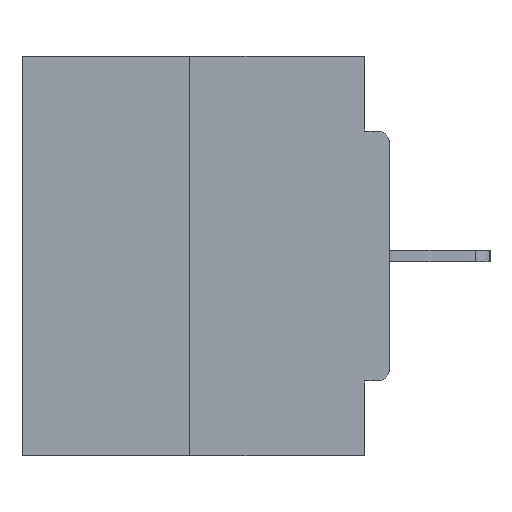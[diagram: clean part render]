
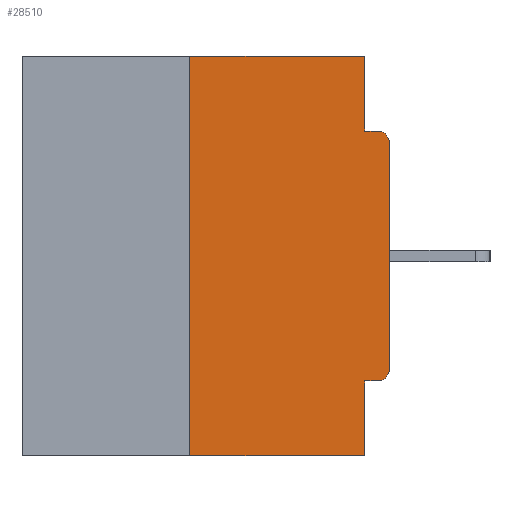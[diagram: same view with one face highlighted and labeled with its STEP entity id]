
A CAD part, left-side view. The second image highlights one B-rep face of the part: STEP entity #28510.
In plain terms, the highlighted planar face has unit normal (-1, 0, 0).
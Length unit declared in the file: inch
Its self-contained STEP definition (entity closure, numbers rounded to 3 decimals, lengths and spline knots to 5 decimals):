
#132 = EDGE_CURVE ( 'NONE', #11339, #19578, #5779, .T. ) ;
#940 = LINE ( 'NONE', #21216, #10678 ) ;
#1049 = LINE ( 'NONE', #2670, #8321 ) ;
#1246 = CARTESIAN_POINT ( 'NONE',  ( 0., 0.015, -0.3915 ) ) ;
#1707 = VECTOR ( 'NONE', #6187, 39.37008 ) ;
#2293 = CARTESIAN_POINT ( 'NONE',  ( 0., 0.25, 0. ) ) ;
#2670 = CARTESIAN_POINT ( 'NONE',  ( 0., 0.25, 0. ) ) ;
#2847 = CARTESIAN_POINT ( 'NONE',  ( 0., 0.015, -0.4065 ) ) ;
#2903 = DIRECTION ( 'NONE',  ( 0., 0., 1. ) ) ;
#3135 = EDGE_CURVE ( 'NONE', #23042, #11339, #20975, .T. ) ;
#3636 = CARTESIAN_POINT ( 'NONE',  ( 0., 0.031, -0.5 ) ) ;
#3715 = CARTESIAN_POINT ( 'NONE',  ( 0., 0.031, 0. ) ) ;
#3979 = ORIENTED_EDGE ( 'NONE', *, *, #6966, .F. ) ;
#4812 = ORIENTED_EDGE ( 'NONE', *, *, #18256, .F. ) ;
#4814 = AXIS2_PLACEMENT_3D ( 'NONE', #7182, #20395, #8969 ) ;
#4815 = CARTESIAN_POINT ( 'NONE',  ( 0., 0.46, 0. ) ) ;
#5355 = DIRECTION ( 'NONE',  ( 0., -1., 0. ) ) ;
#5382 = CARTESIAN_POINT ( 'NONE',  ( 0., 0.46, 0. ) ) ;
#5404 = DIRECTION ( 'NONE',  ( 0., 0., -1. ) ) ;
#5779 = CIRCLE ( 'NONE', #4814, 0.015 ) ;
#6086 = CARTESIAN_POINT ( 'NONE',  ( 0., 0.015, -0.0935 ) ) ;
#6166 = ORIENTED_EDGE ( 'NONE', *, *, #13584, .F. ) ;
#6187 = DIRECTION ( 'NONE',  ( 0., 1., 0. ) ) ;
#6230 = DIRECTION ( 'NONE',  ( 0., 0., -1. ) ) ;
#6966 = EDGE_CURVE ( 'NONE', #11009, #18217, #10561, .T. ) ;
#7108 = CARTESIAN_POINT ( 'NONE',  ( 0., 0.031, -0.0935 ) ) ;
#7182 = CARTESIAN_POINT ( 'NONE',  ( 0., 0.015, -0.1085 ) ) ;
#7282 = VECTOR ( 'NONE', #6230, 39.37008 ) ;
#7327 = FACE_OUTER_BOUND ( 'NONE', #16101, .T. ) ;
#8101 = ORIENTED_EDGE ( 'NONE', *, *, #21871, .T. ) ;
#8168 = ORIENTED_EDGE ( 'NONE', *, *, #21212, .F. ) ;
#8279 = VECTOR ( 'NONE', #24406, 39.37008 ) ;
#8321 = VECTOR ( 'NONE', #22941, 39.37008 ) ;
#8373 = AXIS2_PLACEMENT_3D ( 'NONE', #4815, #16277, #5404 ) ;
#8969 = DIRECTION ( 'NONE',  ( 0., 0., -1. ) ) ;
#10210 = CARTESIAN_POINT ( 'NONE',  ( 0., 0.031, 0. ) ) ;
#10561 = LINE ( 'NONE', #3636, #23821 ) ;
#10594 = VERTEX_POINT ( 'NONE', #2293 ) ;
#10625 = CARTESIAN_POINT ( 'NONE',  ( 0., 0., -0.1085 ) ) ;
#10678 = VECTOR ( 'NONE', #5355, 39.37008 ) ;
#10786 = LINE ( 'NONE', #3715, #7282 ) ;
#11009 = VERTEX_POINT ( 'NONE', #13876 ) ;
#11300 = AXIS2_PLACEMENT_3D ( 'NONE', #1246, #25359, #25495 ) ;
#11339 = VERTEX_POINT ( 'NONE', #10625 ) ;
#11743 = PLANE ( 'NONE',  #8373 ) ;
#13584 = EDGE_CURVE ( 'NONE', #10594, #19589, #25502, .T. ) ;
#13876 = CARTESIAN_POINT ( 'NONE',  ( 0., 0.031, -0.4065 ) ) ;
#14353 = DIRECTION ( 'NONE',  ( 0., -1., 0. ) ) ;
#14930 = ORIENTED_EDGE ( 'NONE', *, *, #3135, .T. ) ;
#15033 = CIRCLE ( 'NONE', #11300, 0.015 ) ;
#16101 = EDGE_LOOP ( 'NONE', ( #6166, #17460, #8101, #3979, #16618, #24232, #14930, #17759, #8168, #4812 ) ) ;
#16277 = DIRECTION ( 'NONE',  ( 1., 0., 0. ) ) ;
#16618 = ORIENTED_EDGE ( 'NONE', *, *, #19889, .F. ) ;
#16737 = VERTEX_POINT ( 'NONE', #26932 ) ;
#17126 = CARTESIAN_POINT ( 'NONE',  ( 0., 0., -0.3915 ) ) ;
#17460 = ORIENTED_EDGE ( 'NONE', *, *, #22278, .F. ) ;
#17759 = ORIENTED_EDGE ( 'NONE', *, *, #132, .T. ) ;
#18217 = VERTEX_POINT ( 'NONE', #22827 ) ;
#18256 = EDGE_CURVE ( 'NONE', #19589, #20950, #10786, .T. ) ;
#19429 = VERTEX_POINT ( 'NONE', #2847 ) ;
#19499 = DIRECTION ( 'NONE',  ( 0., 0., -1. ) ) ;
#19535 = LINE ( 'NONE', #26304, #1707 ) ;
#19578 = VERTEX_POINT ( 'NONE', #6086 ) ;
#19589 = VERTEX_POINT ( 'NONE', #10210 ) ;
#19889 = EDGE_CURVE ( 'NONE', #19429, #11009, #19535, .T. ) ;
#20395 = DIRECTION ( 'NONE',  ( -1., 0., 0. ) ) ;
#20918 = VECTOR ( 'NONE', #2903, 39.37008 ) ;
#20950 = VERTEX_POINT ( 'NONE', #7108 ) ;
#20975 = LINE ( 'NONE', #27600, #20918 ) ;
#21212 = EDGE_CURVE ( 'NONE', #20950, #19578, #22480, .T. ) ;
#21216 = CARTESIAN_POINT ( 'NONE',  ( 0., 0.46, -0.5 ) ) ;
#21871 = EDGE_CURVE ( 'NONE', #16737, #18217, #940, .T. ) ;
#22205 = VECTOR ( 'NONE', #14353, 39.37008 ) ;
#22278 = EDGE_CURVE ( 'NONE', #16737, #10594, #1049, .T. ) ;
#22480 = LINE ( 'NONE', #24253, #8279 ) ;
#22827 = CARTESIAN_POINT ( 'NONE',  ( 0., 0.031, -0.5 ) ) ;
#22941 = DIRECTION ( 'NONE',  ( 0., 0., 1. ) ) ;
#23042 = VERTEX_POINT ( 'NONE', #17126 ) ;
#23821 = VECTOR ( 'NONE', #19499, 39.37008 ) ;
#24232 = ORIENTED_EDGE ( 'NONE', *, *, #26365, .T. ) ;
#24253 = CARTESIAN_POINT ( 'NONE',  ( 0., 0., -0.0935 ) ) ;
#24406 = DIRECTION ( 'NONE',  ( 0., -1., 0. ) ) ;
#25359 = DIRECTION ( 'NONE',  ( -1., 0., 0. ) ) ;
#25495 = DIRECTION ( 'NONE',  ( 0., 0., -1. ) ) ;
#25502 = LINE ( 'NONE', #5382, #22205 ) ;
#26304 = CARTESIAN_POINT ( 'NONE',  ( 0., 0., -0.4065 ) ) ;
#26365 = EDGE_CURVE ( 'NONE', #19429, #23042, #15033, .T. ) ;
#26932 = CARTESIAN_POINT ( 'NONE',  ( 0., 0.25, -0.5 ) ) ;
#27600 = CARTESIAN_POINT ( 'NONE',  ( 0., 0., 0. ) ) ;
#28510 = ADVANCED_FACE ( 'NONE', ( #7327 ), #11743, .F. ) ;
